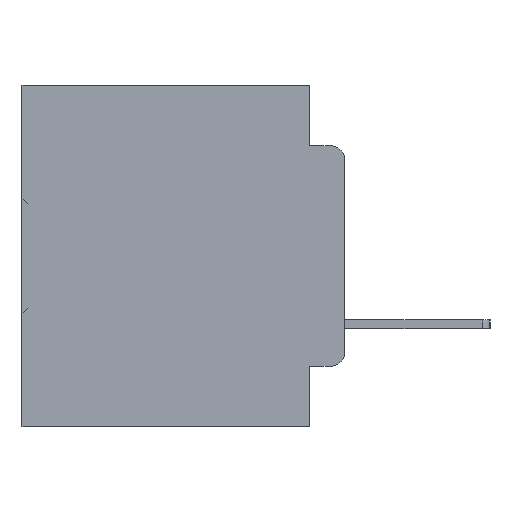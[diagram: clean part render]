
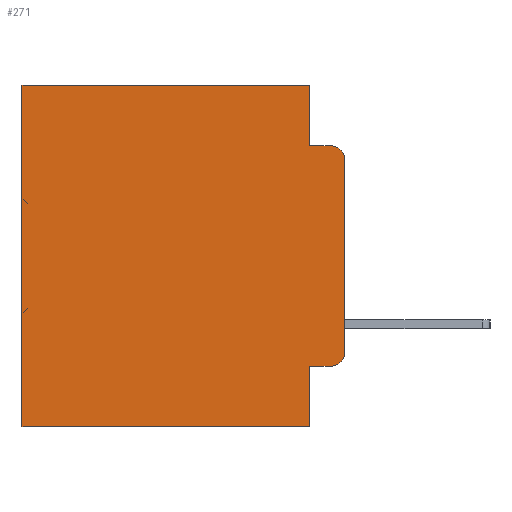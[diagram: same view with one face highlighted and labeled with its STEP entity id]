
A CAD part, left-side view. The second image highlights one B-rep face of the part: STEP entity #271.
In plain terms, the highlighted planar face has unit normal (-1, 0, 0).
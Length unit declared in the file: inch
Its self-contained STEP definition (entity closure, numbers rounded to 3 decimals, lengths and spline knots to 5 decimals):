
#38 = CARTESIAN_POINT ( 'NONE',  ( 0.298, 0.473, 0. ) ) ;
#271 = ADVANCED_FACE ( 'NONE', ( #21128 ), #9179, .F. ) ;
#282 = VERTEX_POINT ( 'NONE', #30291 ) ;
#340 = DIRECTION ( 'NONE',  ( 0., 0., -1. ) ) ;
#356 = ORIENTED_EDGE ( 'NONE', *, *, #35254, .T. ) ;
#544 = CARTESIAN_POINT ( 'NONE',  ( 0.298, 0.473, 0. ) ) ;
#1656 = EDGE_CURVE ( 'NONE', #6506, #34892, #26555, .T. ) ;
#2250 = VERTEX_POINT ( 'NONE', #7299 ) ;
#2638 = AXIS2_PLACEMENT_3D ( 'NONE', #19359, #22134, #5770 ) ;
#2973 = VERTEX_POINT ( 'NONE', #11035 ) ;
#3114 = DIRECTION ( 'NONE',  ( 0., -1., 0. ) ) ;
#3118 = VECTOR ( 'NONE', #35031, 39.37008 ) ;
#3325 = DIRECTION ( 'NONE',  ( 0., 1., 0. ) ) ;
#3557 = VECTOR ( 'NONE', #19182, 39.37008 ) ;
#4011 = LINE ( 'NONE', #25182, #12168 ) ;
#4379 = AXIS2_PLACEMENT_3D ( 'NONE', #9819, #28875, #12573 ) ;
#4426 = VERTEX_POINT ( 'NONE', #18327 ) ;
#4771 = EDGE_CURVE ( 'NONE', #2250, #13176, #4011, .T. ) ;
#5770 = DIRECTION ( 'NONE',  ( 0., 0., -1. ) ) ;
#5789 = LINE ( 'NONE', #11325, #7522 ) ;
#6209 = EDGE_CURVE ( 'NONE', #2250, #4426, #21932, .T. ) ;
#6506 = VERTEX_POINT ( 'NONE', #26245 ) ;
#6628 = ORIENTED_EDGE ( 'NONE', *, *, #34639, .T. ) ;
#6897 = LINE ( 'NONE', #38, #20561 ) ;
#7299 = CARTESIAN_POINT ( 'NONE',  ( 0.298, 0.051, 0. ) ) ;
#7363 = EDGE_CURVE ( 'NONE', #13176, #282, #6897, .T. ) ;
#7522 = VECTOR ( 'NONE', #3114, 39.37008 ) ;
#7813 = VERTEX_POINT ( 'NONE', #34833 ) ;
#9179 = PLANE ( 'NONE',  #2638 ) ;
#9528 = VECTOR ( 'NONE', #18930, 39.37008 ) ;
#9819 = CARTESIAN_POINT ( 'NONE',  ( 0.298, 0.02, -0.3915 ) ) ;
#10039 = ORIENTED_EDGE ( 'NONE', *, *, #4771, .T. ) ;
#11035 = CARTESIAN_POINT ( 'NONE',  ( 0.298, 0., -0.1085 ) ) ;
#11325 = CARTESIAN_POINT ( 'NONE',  ( 0.298, 0.051, -0.0885 ) ) ;
#12118 = LINE ( 'NONE', #21710, #9528 ) ;
#12168 = VECTOR ( 'NONE', #3325, 39.37008 ) ;
#12573 = DIRECTION ( 'NONE',  ( 0., 0., -1. ) ) ;
#13176 = VERTEX_POINT ( 'NONE', #544 ) ;
#14603 = DIRECTION ( 'NONE',  ( -1., 0., 0. ) ) ;
#14637 = VECTOR ( 'NONE', #340, 39.37008 ) ;
#15142 = LINE ( 'NONE', #16118, #3118 ) ;
#15340 = EDGE_CURVE ( 'NONE', #4426, #7813, #5789, .T. ) ;
#15586 = ORIENTED_EDGE ( 'NONE', *, *, #6209, .F. ) ;
#16118 = CARTESIAN_POINT ( 'NONE',  ( 0.298, 0., -0.5 ) ) ;
#16990 = CARTESIAN_POINT ( 'NONE',  ( 0.298, 0.051, 0. ) ) ;
#17288 = ORIENTED_EDGE ( 'NONE', *, *, #7363, .T. ) ;
#17862 = EDGE_CURVE ( 'NONE', #6506, #23272, #25354, .T. ) ;
#18066 = DIRECTION ( 'NONE',  ( 0., -1., 0. ) ) ;
#18327 = CARTESIAN_POINT ( 'NONE',  ( 0.298, 0.051, -0.0885 ) ) ;
#18549 = EDGE_CURVE ( 'NONE', #2973, #28088, #12118, .T. ) ;
#18930 = DIRECTION ( 'NONE',  ( 0., 0., -1. ) ) ;
#19141 = CARTESIAN_POINT ( 'NONE',  ( 0.298, 0.051, -0.5 ) ) ;
#19182 = DIRECTION ( 'NONE',  ( 0., 0., -1. ) ) ;
#19359 = CARTESIAN_POINT ( 'NONE',  ( 0.298, 0., 0. ) ) ;
#19406 = DIRECTION ( 'NONE',  ( 0., 0., -1. ) ) ;
#19860 = ORIENTED_EDGE ( 'NONE', *, *, #17862, .F. ) ;
#20274 = ORIENTED_EDGE ( 'NONE', *, *, #18549, .F. ) ;
#20561 = VECTOR ( 'NONE', #19406, 39.37008 ) ;
#21128 = FACE_OUTER_BOUND ( 'NONE', #26942, .T. ) ;
#21319 = CARTESIAN_POINT ( 'NONE',  ( 0.298, 0.02, -0.4115 ) ) ;
#21710 = CARTESIAN_POINT ( 'NONE',  ( 0.298, 0., 0. ) ) ;
#21932 = LINE ( 'NONE', #16990, #14637 ) ;
#22134 = DIRECTION ( 'NONE',  ( 1., 0., 0. ) ) ;
#22922 = AXIS2_PLACEMENT_3D ( 'NONE', #30920, #14603, #33558 ) ;
#23272 = VERTEX_POINT ( 'NONE', #19141 ) ;
#23757 = EDGE_CURVE ( 'NONE', #23272, #282, #15142, .T. ) ;
#25182 = CARTESIAN_POINT ( 'NONE',  ( 0.298, 0., 0. ) ) ;
#25354 = LINE ( 'NONE', #35212, #3557 ) ;
#26245 = CARTESIAN_POINT ( 'NONE',  ( 0.298, 0.051, -0.4115 ) ) ;
#26555 = LINE ( 'NONE', #34253, #35347 ) ;
#26825 = CIRCLE ( 'NONE', #4379, 0.02 ) ;
#26942 = EDGE_LOOP ( 'NONE', ( #20274, #6628, #29200, #15586, #10039, #17288, #31734, #19860, #34207, #356 ) ) ;
#28088 = VERTEX_POINT ( 'NONE', #30577 ) ;
#28875 = DIRECTION ( 'NONE',  ( -1., 0., 0. ) ) ;
#29200 = ORIENTED_EDGE ( 'NONE', *, *, #15340, .F. ) ;
#30291 = CARTESIAN_POINT ( 'NONE',  ( 0.298, 0.473, -0.5 ) ) ;
#30577 = CARTESIAN_POINT ( 'NONE',  ( 0.298, 0., -0.3915 ) ) ;
#30920 = CARTESIAN_POINT ( 'NONE',  ( 0.298, 0.02, -0.1085 ) ) ;
#31734 = ORIENTED_EDGE ( 'NONE', *, *, #23757, .F. ) ;
#33558 = DIRECTION ( 'NONE',  ( 0., 0., -1. ) ) ;
#34207 = ORIENTED_EDGE ( 'NONE', *, *, #1656, .T. ) ;
#34253 = CARTESIAN_POINT ( 'NONE',  ( 0.298, 0.051, -0.4115 ) ) ;
#34639 = EDGE_CURVE ( 'NONE', #2973, #7813, #35250, .T. ) ;
#34833 = CARTESIAN_POINT ( 'NONE',  ( 0.298, 0.02, -0.0885 ) ) ;
#34892 = VERTEX_POINT ( 'NONE', #21319 ) ;
#35031 = DIRECTION ( 'NONE',  ( 0., 1., 0. ) ) ;
#35212 = CARTESIAN_POINT ( 'NONE',  ( 0.298, 0.051, 0. ) ) ;
#35250 = CIRCLE ( 'NONE', #22922, 0.02 ) ;
#35254 = EDGE_CURVE ( 'NONE', #34892, #28088, #26825, .T. ) ;
#35347 = VECTOR ( 'NONE', #18066, 39.37008 ) ;
